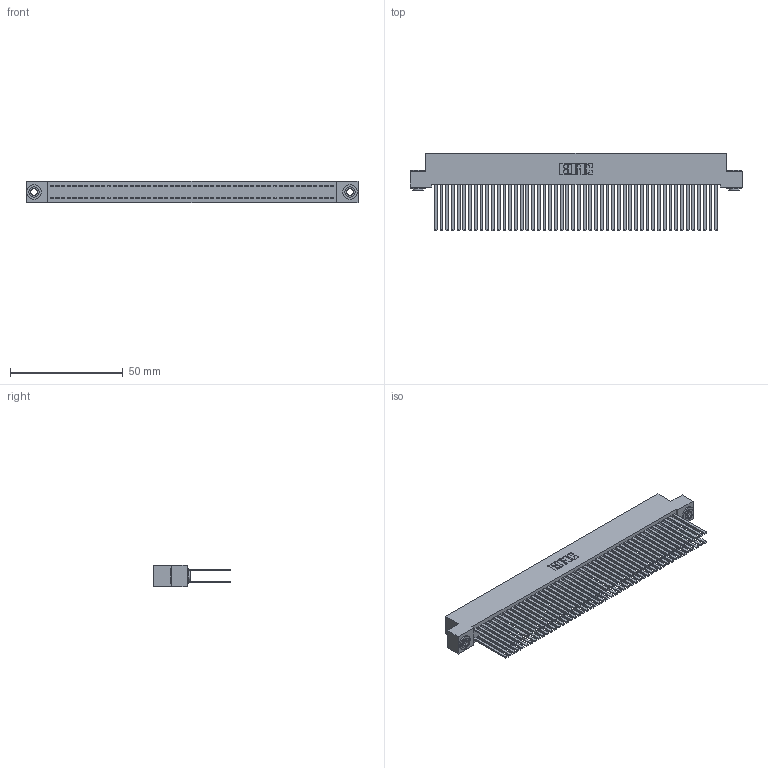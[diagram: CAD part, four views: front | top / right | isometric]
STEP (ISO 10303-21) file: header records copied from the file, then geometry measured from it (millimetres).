
FILE_DESCRIPTION (( 'STEP AP203' ), '1' );
FILE_NAME ('342-100-544-203.STEP', '2019-10-04T17:44:57', ( '' ), ( '' ), 'SwSTEP 2.0', 'SolidWorks 2016', '' );
FILE_SCHEMA (( 'CONFIG_CONTROL_DESIGN' ));
Length unit declared in the file: inch
Products named in the file (4): 342 Part_.156 TH; 345-292-001_345-293-144; 342-250-002_345-250-002-102; 342-100-544-203
Assembly tree (103 placements, depth 2):
  342-100-544-203
    342 Part_.156 TH
    345-292-001_345-293-144  x100
    342-250-002_345-250-002-102  x2
Bounding box: 147.32 x 34.3 x 9.4 mm (x, y, z)
Volume: 14699.2 mm3; surface area: 28219.9 mm2
Topology: 103 solids, 103 shells, 4748 faces, 14075 edges, 9246 vertices
Faces by surface type: plane 3276, cylinder 1464, cone 8
Entity records: 31466 total; most frequent: CARTESIAN_POINT 5177, ORIENTED_EDGE 5106, DIRECTION 4439, EDGE_CURVE 2553, LINE 2405, VECTOR 2405, VERTEX_POINT 1698, AXIS2_PLACEMENT_3D 1017
